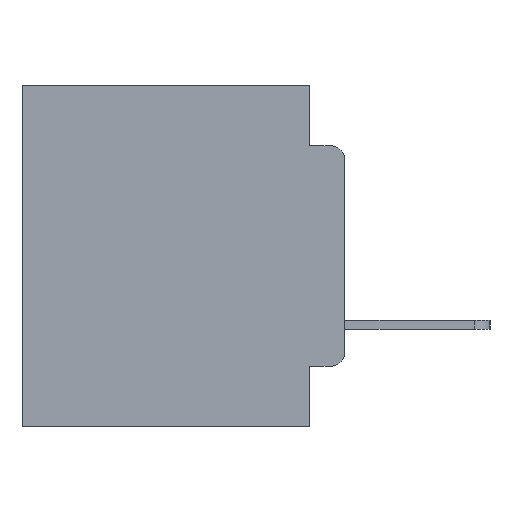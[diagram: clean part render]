
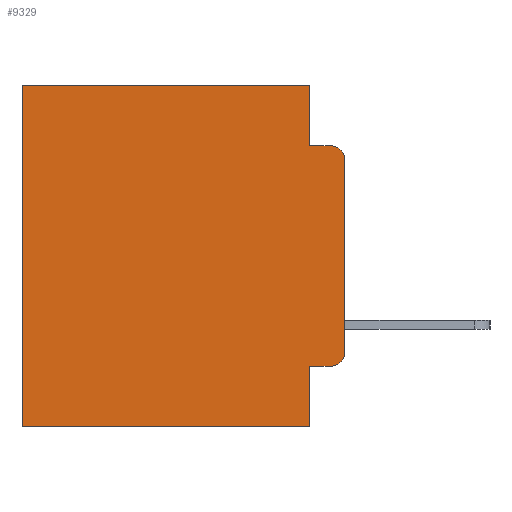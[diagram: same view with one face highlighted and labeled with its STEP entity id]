
A CAD part, left-side view. The second image highlights one B-rep face of the part: STEP entity #9329.
In plain terms, the highlighted planar face has unit normal (-1, 0, 0).
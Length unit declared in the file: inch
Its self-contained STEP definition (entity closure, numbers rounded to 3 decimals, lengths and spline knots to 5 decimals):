
#11 = EDGE_CURVE ( 'NONE', #7885, #26445, #10247, .T. ) ;
#51 = PLANE ( 'NONE',  #11073 ) ;
#252 = CARTESIAN_POINT ( 'NONE',  ( 0.298, 0., -0.1085 ) ) ;
#1346 = FACE_OUTER_BOUND ( 'NONE', #12454, .T. ) ;
#1385 = VERTEX_POINT ( 'NONE', #8347 ) ;
#1882 = CARTESIAN_POINT ( 'NONE',  ( 0.298, 0.473, 0. ) ) ;
#1995 = LINE ( 'NONE', #3253, #18524 ) ;
#2031 = VERTEX_POINT ( 'NONE', #20619 ) ;
#2602 = VECTOR ( 'NONE', #16526, 39.37008 ) ;
#3253 = CARTESIAN_POINT ( 'NONE',  ( 0.298, 0.051, -0.4115 ) ) ;
#3574 = DIRECTION ( 'NONE',  ( 0., 1., 0. ) ) ;
#4073 = VECTOR ( 'NONE', #22091, 39.37008 ) ;
#4396 = VERTEX_POINT ( 'NONE', #11549 ) ;
#4841 = ORIENTED_EDGE ( 'NONE', *, *, #7037, .F. ) ;
#4881 = ORIENTED_EDGE ( 'NONE', *, *, #16133, .T. ) ;
#4895 = DIRECTION ( 'NONE',  ( 0., 0., -1. ) ) ;
#5067 = ORIENTED_EDGE ( 'NONE', *, *, #18318, .F. ) ;
#5103 = CARTESIAN_POINT ( 'NONE',  ( 0.298, 0.051, -0.0885 ) ) ;
#5174 = ORIENTED_EDGE ( 'NONE', *, *, #24243, .F. ) ;
#5283 = ORIENTED_EDGE ( 'NONE', *, *, #9623, .T. ) ;
#5398 = LINE ( 'NONE', #20984, #8531 ) ;
#5485 = ORIENTED_EDGE ( 'NONE', *, *, #23368, .T. ) ;
#5564 = ORIENTED_EDGE ( 'NONE', *, *, #21672, .F. ) ;
#5761 = ORIENTED_EDGE ( 'NONE', *, *, #21780, .F. ) ;
#5784 = ORIENTED_EDGE ( 'NONE', *, *, #22122, .T. ) ;
#5810 = ORIENTED_EDGE ( 'NONE', *, *, #11, .T. ) ;
#5825 = CARTESIAN_POINT ( 'NONE',  ( 0.298, 0., -0.5 ) ) ;
#6338 = VERTEX_POINT ( 'NONE', #252 ) ;
#7037 = EDGE_CURVE ( 'NONE', #6338, #26445, #14951, .T. ) ;
#7327 = DIRECTION ( 'NONE',  ( 0., -1., 0. ) ) ;
#7716 = VECTOR ( 'NONE', #7327, 39.37008 ) ;
#7885 = VERTEX_POINT ( 'NONE', #11598 ) ;
#8347 = CARTESIAN_POINT ( 'NONE',  ( 0.298, 0.02, -0.0885 ) ) ;
#8531 = VECTOR ( 'NONE', #12970, 39.37008 ) ;
#9037 = LINE ( 'NONE', #21570, #23394 ) ;
#9201 = VECTOR ( 'NONE', #23678, 39.37008 ) ;
#9221 = VERTEX_POINT ( 'NONE', #1882 ) ;
#9329 = ADVANCED_FACE ( 'NONE', ( #1346 ), #51, .F. ) ;
#9623 = EDGE_CURVE ( 'NONE', #4396, #9221, #9037, .T. ) ;
#9819 = CARTESIAN_POINT ( 'NONE',  ( 0.298, 0.473, 0. ) ) ;
#10247 = CIRCLE ( 'NONE', #12103, 0.02 ) ;
#11073 = AXIS2_PLACEMENT_3D ( 'NONE', #22130, #19256, #4895 ) ;
#11372 = DIRECTION ( 'NONE',  ( 0., 0., -1. ) ) ;
#11435 = AXIS2_PLACEMENT_3D ( 'NONE', #11602, #12931, #11372 ) ;
#11549 = CARTESIAN_POINT ( 'NONE',  ( 0.298, 0.051, 0. ) ) ;
#11598 = CARTESIAN_POINT ( 'NONE',  ( 0.298, 0.02, -0.4115 ) ) ;
#11602 = CARTESIAN_POINT ( 'NONE',  ( 0.298, 0.02, -0.1085 ) ) ;
#12103 = AXIS2_PLACEMENT_3D ( 'NONE', #19235, #16561, #22384 ) ;
#12443 = VERTEX_POINT ( 'NONE', #23780 ) ;
#12454 = EDGE_LOOP ( 'NONE', ( #4841, #4881, #5067, #5174, #5283, #5485, #5564, #5761, #5784, #5810 ) ) ;
#12746 = VERTEX_POINT ( 'NONE', #14498 ) ;
#12931 = DIRECTION ( 'NONE',  ( -1., 0., 0. ) ) ;
#12970 = DIRECTION ( 'NONE',  ( 0., 0., -1. ) ) ;
#13862 = CIRCLE ( 'NONE', #11435, 0.02 ) ;
#14498 = CARTESIAN_POINT ( 'NONE',  ( 0.298, 0.051, -0.4115 ) ) ;
#14951 = LINE ( 'NONE', #21549, #9201 ) ;
#16133 = EDGE_CURVE ( 'NONE', #6338, #1385, #13862, .T. ) ;
#16258 = DIRECTION ( 'NONE',  ( 0., -1., 0. ) ) ;
#16270 = LINE ( 'NONE', #9819, #4073 ) ;
#16448 = CARTESIAN_POINT ( 'NONE',  ( 0.298, 0.051, -0.5 ) ) ;
#16526 = DIRECTION ( 'NONE',  ( 0., 0., -1. ) ) ;
#16561 = DIRECTION ( 'NONE',  ( -1., 0., 0. ) ) ;
#18318 = EDGE_CURVE ( 'NONE', #12443, #1385, #24025, .T. ) ;
#18524 = VECTOR ( 'NONE', #16258, 39.37008 ) ;
#18538 = CARTESIAN_POINT ( 'NONE',  ( 0.298, 0.051, 0. ) ) ;
#19235 = CARTESIAN_POINT ( 'NONE',  ( 0.298, 0.02, -0.3915 ) ) ;
#19256 = DIRECTION ( 'NONE',  ( 1., 0., 0. ) ) ;
#19608 = VERTEX_POINT ( 'NONE', #16448 ) ;
#20318 = LINE ( 'NONE', #18538, #2602 ) ;
#20619 = CARTESIAN_POINT ( 'NONE',  ( 0.298, 0.473, -0.5 ) ) ;
#20984 = CARTESIAN_POINT ( 'NONE',  ( 0.298, 0.051, 0. ) ) ;
#21289 = DIRECTION ( 'NONE',  ( 0., 1., 0. ) ) ;
#21549 = CARTESIAN_POINT ( 'NONE',  ( 0.298, 0., 0. ) ) ;
#21570 = CARTESIAN_POINT ( 'NONE',  ( 0.298, 0., 0. ) ) ;
#21672 = EDGE_CURVE ( 'NONE', #19608, #2031, #23280, .T. ) ;
#21780 = EDGE_CURVE ( 'NONE', #12746, #19608, #5398, .T. ) ;
#22091 = DIRECTION ( 'NONE',  ( 0., 0., -1. ) ) ;
#22122 = EDGE_CURVE ( 'NONE', #12746, #7885, #1995, .T. ) ;
#22130 = CARTESIAN_POINT ( 'NONE',  ( 0.298, 0., 0. ) ) ;
#22384 = DIRECTION ( 'NONE',  ( 0., 0., -1. ) ) ;
#22691 = VECTOR ( 'NONE', #3574, 39.37008 ) ;
#23280 = LINE ( 'NONE', #5825, #22691 ) ;
#23368 = EDGE_CURVE ( 'NONE', #9221, #2031, #16270, .T. ) ;
#23394 = VECTOR ( 'NONE', #21289, 39.37008 ) ;
#23678 = DIRECTION ( 'NONE',  ( 0., 0., -1. ) ) ;
#23780 = CARTESIAN_POINT ( 'NONE',  ( 0.298, 0.051, -0.0885 ) ) ;
#24025 = LINE ( 'NONE', #5103, #7716 ) ;
#24243 = EDGE_CURVE ( 'NONE', #4396, #12443, #20318, .T. ) ;
#25204 = CARTESIAN_POINT ( 'NONE',  ( 0.298, 0., -0.3915 ) ) ;
#26445 = VERTEX_POINT ( 'NONE', #25204 ) ;
